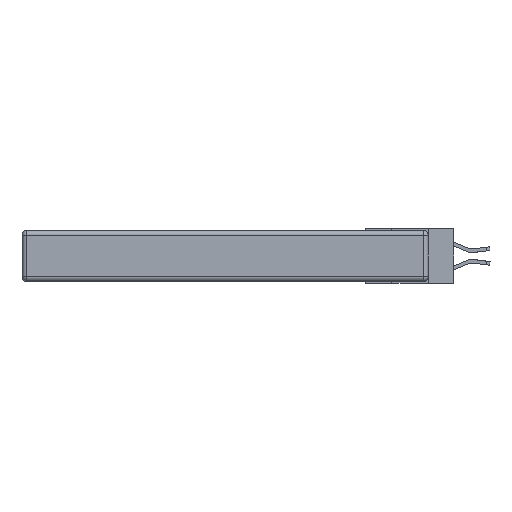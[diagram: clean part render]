
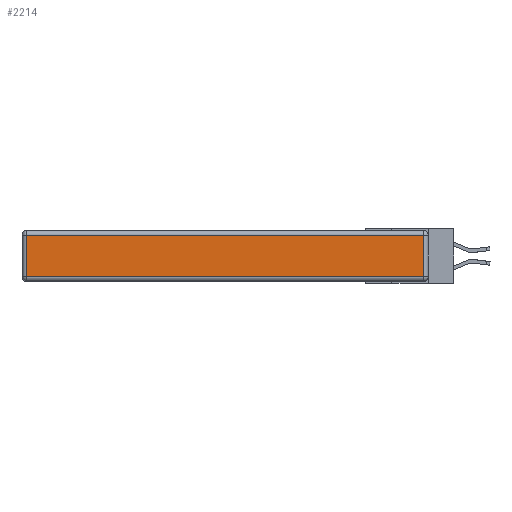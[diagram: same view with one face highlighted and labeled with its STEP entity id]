
A CAD part, left-side view. The second image highlights one B-rep face of the part: STEP entity #2214.
In plain terms, the highlighted planar face has unit normal (-1, 0, 0).
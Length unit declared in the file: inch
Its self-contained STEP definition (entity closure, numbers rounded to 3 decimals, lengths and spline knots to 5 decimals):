
#302 = VERTEX_POINT ( 'NONE', #6874 ) ;
#425 = VECTOR ( 'NONE', #1446, 39.37008 ) ;
#1154 = DIRECTION ( 'NONE',  ( 0., -1., 0. ) ) ;
#1183 = LINE ( 'NONE', #6301, #425 ) ;
#1203 = VECTOR ( 'NONE', #1741, 39.37008 ) ;
#1446 = DIRECTION ( 'NONE',  ( 0., 1., 0. ) ) ;
#1741 = DIRECTION ( 'NONE',  ( 0., 0., -1. ) ) ;
#1896 = AXIS2_PLACEMENT_3D ( 'NONE', #5454, #5412, #7487 ) ;
#2132 = EDGE_CURVE ( 'NONE', #9964, #8388, #8162, .T. ) ;
#2214 = ADVANCED_FACE ( 'NONE', ( #10125 ), #3588, .T. ) ;
#2611 = ORIENTED_EDGE ( 'NONE', *, *, #9977, .T. ) ;
#2996 = LINE ( 'NONE', #12276, #1203 ) ;
#3177 = CARTESIAN_POINT ( 'NONE',  ( 0., 0.03, -0.03 ) ) ;
#3588 = PLANE ( 'NONE',  #1896 ) ;
#4090 = ORIENTED_EDGE ( 'NONE', *, *, #9843, .T. ) ;
#4583 = ORIENTED_EDGE ( 'NONE', *, *, #2132, .T. ) ;
#5245 = CARTESIAN_POINT ( 'NONE',  ( 0., 2.72, -0.313 ) ) ;
#5313 = ORIENTED_EDGE ( 'NONE', *, *, #9393, .T. ) ;
#5412 = DIRECTION ( 'NONE',  ( -1., 0., 0. ) ) ;
#5454 = CARTESIAN_POINT ( 'NONE',  ( 0., 0., -0.343 ) ) ;
#5565 = VECTOR ( 'NONE', #1154, 39.37008 ) ;
#6301 = CARTESIAN_POINT ( 'NONE',  ( 0., 2.75, -0.03 ) ) ;
#6445 = VERTEX_POINT ( 'NONE', #3177 ) ;
#6874 = CARTESIAN_POINT ( 'NONE',  ( 0., 2.72, -0.03 ) ) ;
#7487 = DIRECTION ( 'NONE',  ( 0., 0., 1. ) ) ;
#7793 = CARTESIAN_POINT ( 'NONE',  ( 0., 0.03, -0.343 ) ) ;
#8162 = LINE ( 'NONE', #9068, #5565 ) ;
#8388 = VERTEX_POINT ( 'NONE', #11564 ) ;
#8467 = LINE ( 'NONE', #7793, #12396 ) ;
#9068 = CARTESIAN_POINT ( 'NONE',  ( 0., 0., -0.313 ) ) ;
#9393 = EDGE_CURVE ( 'NONE', #302, #9964, #2996, .T. ) ;
#9843 = EDGE_CURVE ( 'NONE', #8388, #6445, #8467, .T. ) ;
#9964 = VERTEX_POINT ( 'NONE', #5245 ) ;
#9977 = EDGE_CURVE ( 'NONE', #6445, #302, #1183, .T. ) ;
#10125 = FACE_OUTER_BOUND ( 'NONE', #11005, .T. ) ;
#11005 = EDGE_LOOP ( 'NONE', ( #4583, #4090, #2611, #5313 ) ) ;
#11564 = CARTESIAN_POINT ( 'NONE',  ( 0., 0.03, -0.313 ) ) ;
#11696 = DIRECTION ( 'NONE',  ( 0., 0., 1. ) ) ;
#12276 = CARTESIAN_POINT ( 'NONE',  ( 0., 2.72, -0.343 ) ) ;
#12396 = VECTOR ( 'NONE', #11696, 39.37008 ) ;
